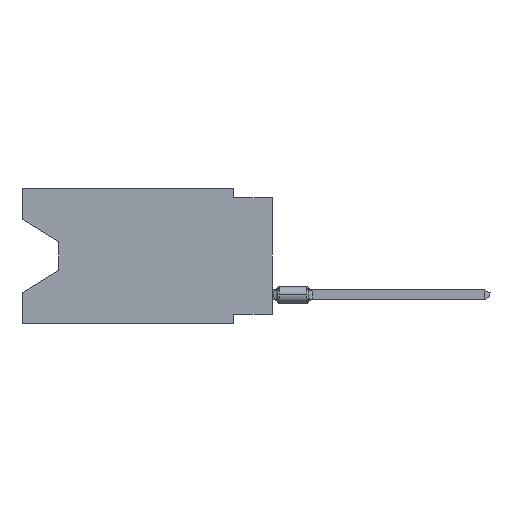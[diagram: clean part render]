
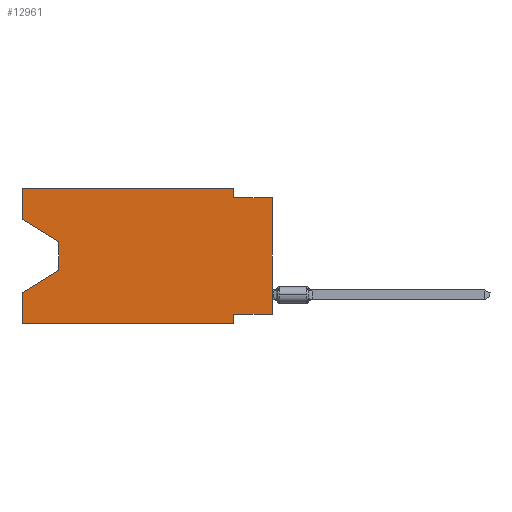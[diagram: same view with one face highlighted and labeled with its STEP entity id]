
A CAD part, left-side view. The second image highlights one B-rep face of the part: STEP entity #12961.
In plain terms, the highlighted planar face has unit normal (-1, 0, 0).
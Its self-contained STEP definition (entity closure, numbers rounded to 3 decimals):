
#246 = VECTOR ( 'NONE', #32528, 1000. ) ;
#908 = CARTESIAN_POINT ( 'NONE',  ( 0., 16.383, 0. ) ) ;
#957 = CARTESIAN_POINT ( 'NONE',  ( 0., 0., -8.255 ) ) ;
#2011 = DIRECTION ( 'NONE',  ( 0., 0., -1. ) ) ;
#2524 = LINE ( 'NONE', #31020, #7443 ) ;
#2756 = DIRECTION ( 'NONE',  ( 0., -0.855, -0.519 ) ) ;
#3095 = EDGE_CURVE ( 'NONE', #33163, #5533, #5798, .T. ) ;
#3157 = CARTESIAN_POINT ( 'NONE',  ( 0., 0., -0.635 ) ) ;
#3918 = CARTESIAN_POINT ( 'NONE',  ( 0., 2.54, 0. ) ) ;
#5123 = VERTEX_POINT ( 'NONE', #13989 ) ;
#5266 = DIRECTION ( 'NONE',  ( 0., 0., 1. ) ) ;
#5416 = EDGE_CURVE ( 'NONE', #11832, #24459, #18785, .T. ) ;
#5467 = CARTESIAN_POINT ( 'NONE',  ( 0., 16.383, 0. ) ) ;
#5533 = VERTEX_POINT ( 'NONE', #3918 ) ;
#5663 = EDGE_CURVE ( 'NONE', #11220, #14762, #15266, .T. ) ;
#5754 = VECTOR ( 'NONE', #28081, 1000. ) ;
#5798 = LINE ( 'NONE', #27124, #246 ) ;
#5996 = CARTESIAN_POINT ( 'NONE',  ( 0., 16.383, -8.89 ) ) ;
#6203 = DIRECTION ( 'NONE',  ( 0., 1., 0. ) ) ;
#6846 = VERTEX_POINT ( 'NONE', #5996 ) ;
#7104 = DIRECTION ( 'NONE',  ( 0., -1., 0. ) ) ;
#7443 = VECTOR ( 'NONE', #2011, 1000. ) ;
#7812 = VERTEX_POINT ( 'NONE', #31007 ) ;
#8245 = ORIENTED_EDGE ( 'NONE', *, *, #23361, .F. ) ;
#8250 = PLANE ( 'NONE',  #14060 ) ;
#8269 = EDGE_CURVE ( 'NONE', #11832, #11220, #32753, .T. ) ;
#8427 = VERTEX_POINT ( 'NONE', #20512 ) ;
#8956 = VECTOR ( 'NONE', #7104, 1000. ) ;
#9203 = CARTESIAN_POINT ( 'NONE',  ( 0., 16.383, -6.852 ) ) ;
#9256 = ORIENTED_EDGE ( 'NONE', *, *, #31344, .T. ) ;
#10176 = VECTOR ( 'NONE', #2756, 1000. ) ;
#10531 = CARTESIAN_POINT ( 'NONE',  ( 0., 2.54, -8.89 ) ) ;
#11016 = LINE ( 'NONE', #3157, #8956 ) ;
#11056 = EDGE_LOOP ( 'NONE', ( #13162, #16585, #9256, #8245, #27740, #33883, #12569, #28128, #29375, #22528, #23052, #25898 ) ) ;
#11220 = VERTEX_POINT ( 'NONE', #30342 ) ;
#11315 = CARTESIAN_POINT ( 'NONE',  ( 0., 2.54, 0. ) ) ;
#11426 = VECTOR ( 'NONE', #19132, 1000. ) ;
#11573 = DIRECTION ( 'NONE',  ( 1., 0., 0. ) ) ;
#11832 = VERTEX_POINT ( 'NONE', #32184 ) ;
#12430 = VECTOR ( 'NONE', #26694, 1000. ) ;
#12569 = ORIENTED_EDGE ( 'NONE', *, *, #8269, .F. ) ;
#12961 = ADVANCED_FACE ( 'NONE', ( #14354 ), #8250, .F. ) ;
#13140 = CARTESIAN_POINT ( 'NONE',  ( 0., 16.383, 0. ) ) ;
#13162 = ORIENTED_EDGE ( 'NONE', *, *, #30481, .T. ) ;
#13267 = CARTESIAN_POINT ( 'NONE',  ( 0., 2.54, -8.89 ) ) ;
#13688 = DIRECTION ( 'NONE',  ( 0., 0., 1. ) ) ;
#13989 = CARTESIAN_POINT ( 'NONE',  ( 0., 13.97, -5.385 ) ) ;
#14060 = AXIS2_PLACEMENT_3D ( 'NONE', #908, #11573, #32190 ) ;
#14354 = FACE_OUTER_BOUND ( 'NONE', #11056, .T. ) ;
#14387 = CARTESIAN_POINT ( 'NONE',  ( 0., 16.383, 0. ) ) ;
#14762 = VERTEX_POINT ( 'NONE', #13267 ) ;
#15266 = LINE ( 'NONE', #10531, #25383 ) ;
#15940 = DIRECTION ( 'NONE',  ( 0., -1., 0. ) ) ;
#15993 = EDGE_CURVE ( 'NONE', #7812, #33163, #18537, .T. ) ;
#16027 = LINE ( 'NONE', #11315, #12430 ) ;
#16585 = ORIENTED_EDGE ( 'NONE', *, *, #31786, .T. ) ;
#16685 = CARTESIAN_POINT ( 'NONE',  ( 0., 0., 0. ) ) ;
#17852 = VECTOR ( 'NONE', #5266, 1000. ) ;
#18212 = LINE ( 'NONE', #20843, #27384 ) ;
#18537 = LINE ( 'NONE', #13140, #17852 ) ;
#18737 = LINE ( 'NONE', #5467, #21213 ) ;
#18785 = LINE ( 'NONE', #16685, #11426 ) ;
#19132 = DIRECTION ( 'NONE',  ( 0., 0., 1. ) ) ;
#19855 = CARTESIAN_POINT ( 'NONE',  ( 0., 13.97, -5.385 ) ) ;
#20512 = CARTESIAN_POINT ( 'NONE',  ( 0., 13.97, -3.505 ) ) ;
#20843 = CARTESIAN_POINT ( 'NONE',  ( 0., 16.383, -8.89 ) ) ;
#21213 = VECTOR ( 'NONE', #13688, 1000. ) ;
#22528 = ORIENTED_EDGE ( 'NONE', *, *, #31144, .F. ) ;
#23052 = ORIENTED_EDGE ( 'NONE', *, *, #3095, .F. ) ;
#23361 = EDGE_CURVE ( 'NONE', #6846, #25841, #18737, .T. ) ;
#23889 = EDGE_CURVE ( 'NONE', #25491, #24459, #11016, .T. ) ;
#24459 = VERTEX_POINT ( 'NONE', #30999 ) ;
#25098 = LINE ( 'NONE', #19855, #5754 ) ;
#25383 = VECTOR ( 'NONE', #28388, 1000. ) ;
#25491 = VERTEX_POINT ( 'NONE', #32471 ) ;
#25841 = VERTEX_POINT ( 'NONE', #9203 ) ;
#25898 = ORIENTED_EDGE ( 'NONE', *, *, #15993, .F. ) ;
#26694 = DIRECTION ( 'NONE',  ( 0., 0., -1. ) ) ;
#27124 = CARTESIAN_POINT ( 'NONE',  ( 0., 16.383, 0. ) ) ;
#27384 = VECTOR ( 'NONE', #15940, 1000. ) ;
#27740 = ORIENTED_EDGE ( 'NONE', *, *, #28742, .T. ) ;
#28081 = DIRECTION ( 'NONE',  ( 0., 0.855, -0.519 ) ) ;
#28128 = ORIENTED_EDGE ( 'NONE', *, *, #5416, .T. ) ;
#28388 = DIRECTION ( 'NONE',  ( 0., 0., -1. ) ) ;
#28742 = EDGE_CURVE ( 'NONE', #6846, #14762, #18212, .T. ) ;
#29375 = ORIENTED_EDGE ( 'NONE', *, *, #23889, .F. ) ;
#30342 = CARTESIAN_POINT ( 'NONE',  ( 0., 2.54, -8.255 ) ) ;
#30481 = EDGE_CURVE ( 'NONE', #7812, #8427, #32634, .T. ) ;
#30999 = CARTESIAN_POINT ( 'NONE',  ( 0., 0., -0.635 ) ) ;
#31007 = CARTESIAN_POINT ( 'NONE',  ( 0., 16.383, -2.038 ) ) ;
#31020 = CARTESIAN_POINT ( 'NONE',  ( 0., 13.97, -3.505 ) ) ;
#31144 = EDGE_CURVE ( 'NONE', #5533, #25491, #16027, .T. ) ;
#31344 = EDGE_CURVE ( 'NONE', #5123, #25841, #25098, .T. ) ;
#31786 = EDGE_CURVE ( 'NONE', #8427, #5123, #2524, .T. ) ;
#32106 = CARTESIAN_POINT ( 'NONE',  ( 0., 16.383, -2.038 ) ) ;
#32184 = CARTESIAN_POINT ( 'NONE',  ( 0., 0., -8.255 ) ) ;
#32190 = DIRECTION ( 'NONE',  ( 0., 0., -1. ) ) ;
#32471 = CARTESIAN_POINT ( 'NONE',  ( 0., 2.54, -0.635 ) ) ;
#32528 = DIRECTION ( 'NONE',  ( 0., -1., 0. ) ) ;
#32634 = LINE ( 'NONE', #32106, #10176 ) ;
#32753 = LINE ( 'NONE', #957, #33164 ) ;
#33163 = VERTEX_POINT ( 'NONE', #14387 ) ;
#33164 = VECTOR ( 'NONE', #6203, 1000. ) ;
#33883 = ORIENTED_EDGE ( 'NONE', *, *, #5663, .F. ) ;
